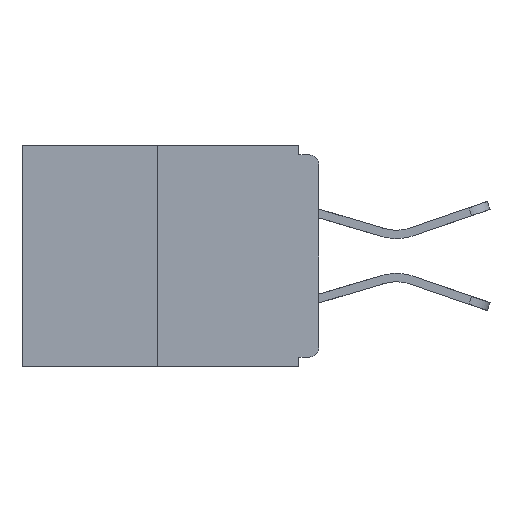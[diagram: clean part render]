
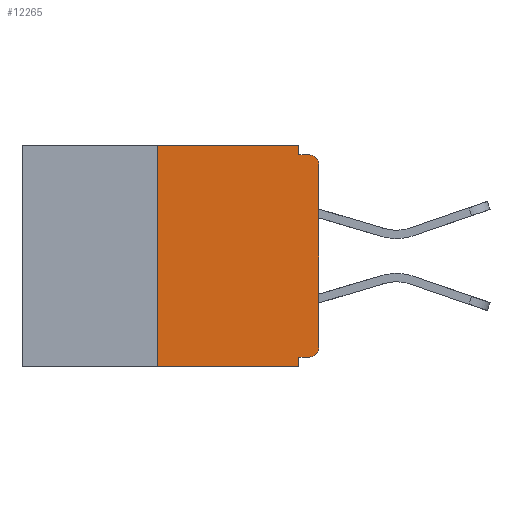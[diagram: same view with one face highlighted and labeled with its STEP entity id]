
A CAD part, left-side view. The second image highlights one B-rep face of the part: STEP entity #12265.
In plain terms, the highlighted planar face has unit normal (-1, 0, 0).
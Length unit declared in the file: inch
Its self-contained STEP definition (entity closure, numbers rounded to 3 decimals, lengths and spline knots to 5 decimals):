
#49 = VECTOR ( 'NONE', #4358, 39.37008 ) ;
#191 = CARTESIAN_POINT ( 'NONE',  ( 0., 0.031, -0.343 ) ) ;
#193 = CIRCLE ( 'NONE', #1652, 0.015 ) ;
#463 = ORIENTED_EDGE ( 'NONE', *, *, #8932, .F. ) ;
#524 = VECTOR ( 'NONE', #13915, 39.37008 ) ;
#565 = DIRECTION ( 'NONE',  ( 0., 0., 1. ) ) ;
#770 = LINE ( 'NONE', #7650, #14734 ) ;
#1301 = VERTEX_POINT ( 'NONE', #12590 ) ;
#1308 = PLANE ( 'NONE',  #7679 ) ;
#1321 = EDGE_CURVE ( 'NONE', #6074, #6775, #3109, .T. ) ;
#1349 = VERTEX_POINT ( 'NONE', #1547 ) ;
#1545 = DIRECTION ( 'NONE',  ( 0., 0., -1. ) ) ;
#1547 = CARTESIAN_POINT ( 'NONE',  ( 0., 0.25, 0. ) ) ;
#1627 = CARTESIAN_POINT ( 'NONE',  ( 0., 0.031, -0.343 ) ) ;
#1652 = AXIS2_PLACEMENT_3D ( 'NONE', #1696, #10670, #14797 ) ;
#1693 = CARTESIAN_POINT ( 'NONE',  ( 0., 0.46, 0. ) ) ;
#1696 = CARTESIAN_POINT ( 'NONE',  ( 0., 0.015, -0.313 ) ) ;
#1825 = CARTESIAN_POINT ( 'NONE',  ( 0., 0., -0.313 ) ) ;
#1955 = CARTESIAN_POINT ( 'NONE',  ( 0., 0.031, 0. ) ) ;
#2054 = ORIENTED_EDGE ( 'NONE', *, *, #2292, .F. ) ;
#2292 = EDGE_CURVE ( 'NONE', #1301, #2720, #7690, .T. ) ;
#2720 = VERTEX_POINT ( 'NONE', #191 ) ;
#2920 = CARTESIAN_POINT ( 'NONE',  ( 0., 0., 0. ) ) ;
#2971 = CARTESIAN_POINT ( 'NONE',  ( 0., 0.031, -0.015 ) ) ;
#3102 = CARTESIAN_POINT ( 'NONE',  ( 0., 0.031, 0. ) ) ;
#3109 = LINE ( 'NONE', #10039, #524 ) ;
#3135 = ORIENTED_EDGE ( 'NONE', *, *, #12405, .T. ) ;
#3938 = ORIENTED_EDGE ( 'NONE', *, *, #1321, .F. ) ;
#4006 = DIRECTION ( 'NONE',  ( 0., -1., 0. ) ) ;
#4358 = DIRECTION ( 'NONE',  ( 0., -1., 0. ) ) ;
#4673 = VECTOR ( 'NONE', #4006, 39.37008 ) ;
#4685 = CARTESIAN_POINT ( 'NONE',  ( 0., 0., -0.03 ) ) ;
#4842 = LINE ( 'NONE', #1693, #49 ) ;
#5219 = EDGE_CURVE ( 'NONE', #10541, #6775, #16304, .T. ) ;
#5914 = ORIENTED_EDGE ( 'NONE', *, *, #14639, .T. ) ;
#6074 = VERTEX_POINT ( 'NONE', #2971 ) ;
#6092 = DIRECTION ( 'NONE',  ( -1., 0., 0. ) ) ;
#6179 = VECTOR ( 'NONE', #9477, 39.37008 ) ;
#6204 = VECTOR ( 'NONE', #12163, 39.37008 ) ;
#6769 = DIRECTION ( 'NONE',  ( 0., 0., -1. ) ) ;
#6775 = VERTEX_POINT ( 'NONE', #12865 ) ;
#7028 = ORIENTED_EDGE ( 'NONE', *, *, #13122, .F. ) ;
#7392 = ORIENTED_EDGE ( 'NONE', *, *, #10803, .F. ) ;
#7531 = LINE ( 'NONE', #10760, #15716 ) ;
#7650 = CARTESIAN_POINT ( 'NONE',  ( 0., 0., -0.328 ) ) ;
#7679 = AXIS2_PLACEMENT_3D ( 'NONE', #14197, #10246, #1545 ) ;
#7690 = LINE ( 'NONE', #1627, #11273 ) ;
#7972 = VERTEX_POINT ( 'NONE', #1825 ) ;
#8390 = AXIS2_PLACEMENT_3D ( 'NONE', #16528, #6092, #8916 ) ;
#8652 = EDGE_LOOP ( 'NONE', ( #7028, #7392, #3135, #2054, #16097, #15685, #5914, #10358, #3938, #463 ) ) ;
#8916 = DIRECTION ( 'NONE',  ( 0., 0., -1. ) ) ;
#8932 = EDGE_CURVE ( 'NONE', #12482, #6074, #16203, .T. ) ;
#9477 = DIRECTION ( 'NONE',  ( 0., 0., 1. ) ) ;
#9678 = EDGE_CURVE ( 'NONE', #11472, #7972, #193, .T. ) ;
#10039 = CARTESIAN_POINT ( 'NONE',  ( 0., 0., -0.015 ) ) ;
#10246 = DIRECTION ( 'NONE',  ( 1., 0., 0. ) ) ;
#10263 = LINE ( 'NONE', #11757, #4673 ) ;
#10358 = ORIENTED_EDGE ( 'NONE', *, *, #5219, .T. ) ;
#10541 = VERTEX_POINT ( 'NONE', #4685 ) ;
#10670 = DIRECTION ( 'NONE',  ( -1., 0., 0. ) ) ;
#10760 = CARTESIAN_POINT ( 'NONE',  ( 0., 0.25, 0. ) ) ;
#10803 = EDGE_CURVE ( 'NONE', #16523, #1349, #7531, .T. ) ;
#11273 = VECTOR ( 'NONE', #6769, 39.37008 ) ;
#11472 = VERTEX_POINT ( 'NONE', #15482 ) ;
#11649 = FACE_OUTER_BOUND ( 'NONE', #8652, .T. ) ;
#11655 = DIRECTION ( 'NONE',  ( 0., 1., 0. ) ) ;
#11757 = CARTESIAN_POINT ( 'NONE',  ( 0., 0.46, -0.343 ) ) ;
#12163 = DIRECTION ( 'NONE',  ( 0., 0., -1. ) ) ;
#12265 = ADVANCED_FACE ( 'NONE', ( #11649 ), #1308, .F. ) ;
#12405 = EDGE_CURVE ( 'NONE', #16523, #2720, #10263, .T. ) ;
#12482 = VERTEX_POINT ( 'NONE', #3102 ) ;
#12590 = CARTESIAN_POINT ( 'NONE',  ( 0., 0.031, -0.328 ) ) ;
#12865 = CARTESIAN_POINT ( 'NONE',  ( 0., 0.015, -0.015 ) ) ;
#12949 = CARTESIAN_POINT ( 'NONE',  ( 0., 0.25, -0.343 ) ) ;
#13122 = EDGE_CURVE ( 'NONE', #1349, #12482, #4842, .T. ) ;
#13915 = DIRECTION ( 'NONE',  ( 0., -1., 0. ) ) ;
#14197 = CARTESIAN_POINT ( 'NONE',  ( 0., 0.46, 0. ) ) ;
#14639 = EDGE_CURVE ( 'NONE', #7972, #10541, #14769, .T. ) ;
#14734 = VECTOR ( 'NONE', #11655, 39.37008 ) ;
#14769 = LINE ( 'NONE', #2920, #6179 ) ;
#14797 = DIRECTION ( 'NONE',  ( 0., 0., -1. ) ) ;
#15482 = CARTESIAN_POINT ( 'NONE',  ( 0., 0.015, -0.328 ) ) ;
#15685 = ORIENTED_EDGE ( 'NONE', *, *, #9678, .T. ) ;
#15716 = VECTOR ( 'NONE', #565, 39.37008 ) ;
#15729 = EDGE_CURVE ( 'NONE', #11472, #1301, #770, .T. ) ;
#16097 = ORIENTED_EDGE ( 'NONE', *, *, #15729, .F. ) ;
#16203 = LINE ( 'NONE', #1955, #6204 ) ;
#16304 = CIRCLE ( 'NONE', #8390, 0.015 ) ;
#16523 = VERTEX_POINT ( 'NONE', #12949 ) ;
#16528 = CARTESIAN_POINT ( 'NONE',  ( 0., 0.015, -0.03 ) ) ;
